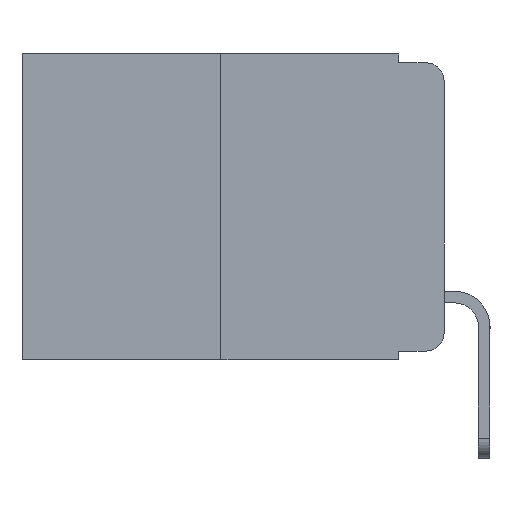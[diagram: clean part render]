
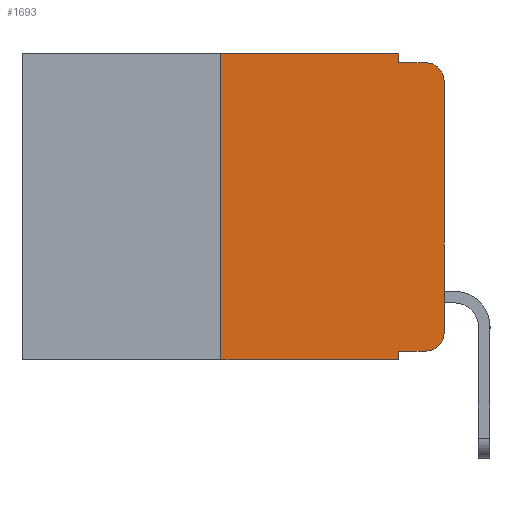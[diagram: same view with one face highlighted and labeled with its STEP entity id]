
A CAD part, left-side view. The second image highlights one B-rep face of the part: STEP entity #1693.
In plain terms, the highlighted planar face has unit normal (-1, 0, 0).
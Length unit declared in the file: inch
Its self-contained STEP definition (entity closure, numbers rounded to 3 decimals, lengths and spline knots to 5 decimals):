
#25 = VECTOR ( 'NONE', #10554, 39.37008 ) ;
#278 = EDGE_CURVE ( 'NONE', #6377, #7715, #7916, .T. ) ;
#357 = ORIENTED_EDGE ( 'NONE', *, *, #278, .F. ) ;
#625 = CARTESIAN_POINT ( 'NONE',  ( 0., 0.051, 0. ) ) ;
#713 = VERTEX_POINT ( 'NONE', #6107 ) ;
#815 = LINE ( 'NONE', #11361, #9017 ) ;
#929 = DIRECTION ( 'NONE',  ( 1., 0., 0. ) ) ;
#1005 = VECTOR ( 'NONE', #5092, 39.37008 ) ;
#1399 = CARTESIAN_POINT ( 'NONE',  ( 0., 0.473, 0. ) ) ;
#1403 = CARTESIAN_POINT ( 'NONE',  ( 0., 0.473, 0. ) ) ;
#1462 = EDGE_CURVE ( 'NONE', #11603, #7766, #10426, .T. ) ;
#1471 = CARTESIAN_POINT ( 'NONE',  ( 0., 0.25, -0.343 ) ) ;
#1693 = ADVANCED_FACE ( 'NONE', ( #4434 ), #8057, .F. ) ;
#1705 = CARTESIAN_POINT ( 'NONE',  ( 0., 0.051, -0.333 ) ) ;
#1789 = VERTEX_POINT ( 'NONE', #5496 ) ;
#1802 = LINE ( 'NONE', #5058, #1005 ) ;
#2187 = VERTEX_POINT ( 'NONE', #4004 ) ;
#2419 = VERTEX_POINT ( 'NONE', #4269 ) ;
#2450 = DIRECTION ( 'NONE',  ( -1., 0., 0. ) ) ;
#2740 = CARTESIAN_POINT ( 'NONE',  ( 0., 0.051, 0. ) ) ;
#2858 = DIRECTION ( 'NONE',  ( 0., -1., 0. ) ) ;
#2868 = AXIS2_PLACEMENT_3D ( 'NONE', #1399, #929, #12038 ) ;
#2994 = EDGE_CURVE ( 'NONE', #7715, #9522, #12420, .T. ) ;
#3064 = LINE ( 'NONE', #625, #13255 ) ;
#3410 = DIRECTION ( 'NONE',  ( 0., -1., 0. ) ) ;
#3828 = CARTESIAN_POINT ( 'NONE',  ( 0., 0.25, 0. ) ) ;
#3893 = ORIENTED_EDGE ( 'NONE', *, *, #4579, .T. ) ;
#3908 = VERTEX_POINT ( 'NONE', #10708 ) ;
#4004 = CARTESIAN_POINT ( 'NONE',  ( 0., 0.051, -0.01 ) ) ;
#4269 = CARTESIAN_POINT ( 'NONE',  ( 0., 0.051, -0.343 ) ) ;
#4368 = VECTOR ( 'NONE', #12607, 39.37008 ) ;
#4434 = FACE_OUTER_BOUND ( 'NONE', #5621, .T. ) ;
#4484 = EDGE_CURVE ( 'NONE', #2187, #3908, #10239, .T. ) ;
#4496 = ORIENTED_EDGE ( 'NONE', *, *, #9793, .T. ) ;
#4579 = EDGE_CURVE ( 'NONE', #1789, #11603, #5506, .T. ) ;
#4624 = ORIENTED_EDGE ( 'NONE', *, *, #1462, .T. ) ;
#4718 = CARTESIAN_POINT ( 'NONE',  ( 0., 0.051, 0. ) ) ;
#5032 = EDGE_CURVE ( 'NONE', #9522, #2187, #8430, .T. ) ;
#5058 = CARTESIAN_POINT ( 'NONE',  ( 0., 0., 0. ) ) ;
#5092 = DIRECTION ( 'NONE',  ( 0., 0., 1. ) ) ;
#5496 = CARTESIAN_POINT ( 'NONE',  ( 0., 0.051, -0.333 ) ) ;
#5506 = LINE ( 'NONE', #1705, #12842 ) ;
#5621 = EDGE_LOOP ( 'NONE', ( #6752, #4496, #7111, #8828, #11577, #357, #6364, #11525, #3893, #4624 ) ) ;
#5947 = EDGE_CURVE ( 'NONE', #1789, #2419, #3064, .T. ) ;
#6107 = CARTESIAN_POINT ( 'NONE',  ( 0., 0., -0.03 ) ) ;
#6364 = ORIENTED_EDGE ( 'NONE', *, *, #10510, .T. ) ;
#6377 = VERTEX_POINT ( 'NONE', #1471 ) ;
#6752 = ORIENTED_EDGE ( 'NONE', *, *, #11621, .T. ) ;
#7111 = ORIENTED_EDGE ( 'NONE', *, *, #4484, .F. ) ;
#7164 = CARTESIAN_POINT ( 'NONE',  ( 0., 0.02, -0.313 ) ) ;
#7381 = DIRECTION ( 'NONE',  ( -1., 0., 0. ) ) ;
#7715 = VERTEX_POINT ( 'NONE', #12241 ) ;
#7766 = VERTEX_POINT ( 'NONE', #13224 ) ;
#7830 = CARTESIAN_POINT ( 'NONE',  ( 0., 0.051, -0.01 ) ) ;
#7916 = LINE ( 'NONE', #3828, #10199 ) ;
#8057 = PLANE ( 'NONE',  #2868 ) ;
#8430 = LINE ( 'NONE', #4718, #25 ) ;
#8706 = CARTESIAN_POINT ( 'NONE',  ( 0., 0.02, -0.03 ) ) ;
#8828 = ORIENTED_EDGE ( 'NONE', *, *, #5032, .F. ) ;
#9017 = VECTOR ( 'NONE', #3410, 39.37008 ) ;
#9251 = DIRECTION ( 'NONE',  ( 0., 0., -1. ) ) ;
#9390 = CIRCLE ( 'NONE', #11791, 0.02 ) ;
#9522 = VERTEX_POINT ( 'NONE', #2740 ) ;
#9660 = DIRECTION ( 'NONE',  ( 0., 0., -1. ) ) ;
#9793 = EDGE_CURVE ( 'NONE', #713, #3908, #9390, .T. ) ;
#10007 = DIRECTION ( 'NONE',  ( 0., 0., 1. ) ) ;
#10199 = VECTOR ( 'NONE', #10007, 39.37008 ) ;
#10207 = AXIS2_PLACEMENT_3D ( 'NONE', #7164, #7381, #11123 ) ;
#10239 = LINE ( 'NONE', #7830, #4368 ) ;
#10426 = CIRCLE ( 'NONE', #10207, 0.02 ) ;
#10510 = EDGE_CURVE ( 'NONE', #6377, #2419, #815, .T. ) ;
#10554 = DIRECTION ( 'NONE',  ( 0., 0., -1. ) ) ;
#10708 = CARTESIAN_POINT ( 'NONE',  ( 0., 0.02, -0.01 ) ) ;
#11123 = DIRECTION ( 'NONE',  ( 0., 0., -1. ) ) ;
#11361 = CARTESIAN_POINT ( 'NONE',  ( 0., 0.473, -0.343 ) ) ;
#11525 = ORIENTED_EDGE ( 'NONE', *, *, #5947, .F. ) ;
#11577 = ORIENTED_EDGE ( 'NONE', *, *, #2994, .F. ) ;
#11603 = VERTEX_POINT ( 'NONE', #12685 ) ;
#11621 = EDGE_CURVE ( 'NONE', #7766, #713, #1802, .T. ) ;
#11624 = DIRECTION ( 'NONE',  ( 0., -1., 0. ) ) ;
#11791 = AXIS2_PLACEMENT_3D ( 'NONE', #8706, #2450, #9660 ) ;
#12038 = DIRECTION ( 'NONE',  ( 0., 0., -1. ) ) ;
#12125 = VECTOR ( 'NONE', #11624, 39.37008 ) ;
#12241 = CARTESIAN_POINT ( 'NONE',  ( 0., 0.25, 0. ) ) ;
#12420 = LINE ( 'NONE', #1403, #12125 ) ;
#12607 = DIRECTION ( 'NONE',  ( 0., -1., 0. ) ) ;
#12685 = CARTESIAN_POINT ( 'NONE',  ( 0., 0.02, -0.333 ) ) ;
#12842 = VECTOR ( 'NONE', #2858, 39.37008 ) ;
#13224 = CARTESIAN_POINT ( 'NONE',  ( 0., 0., -0.313 ) ) ;
#13255 = VECTOR ( 'NONE', #9251, 39.37008 ) ;
